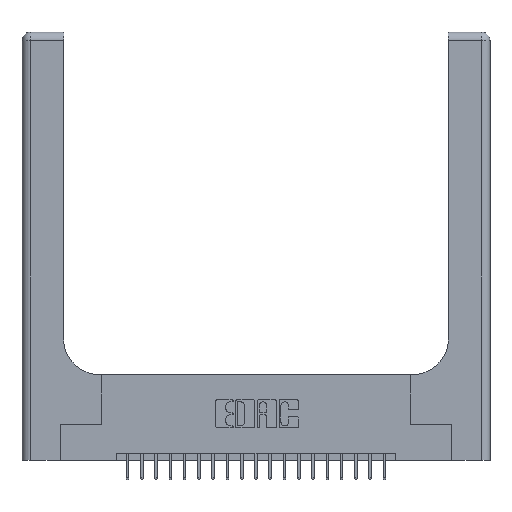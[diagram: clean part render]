
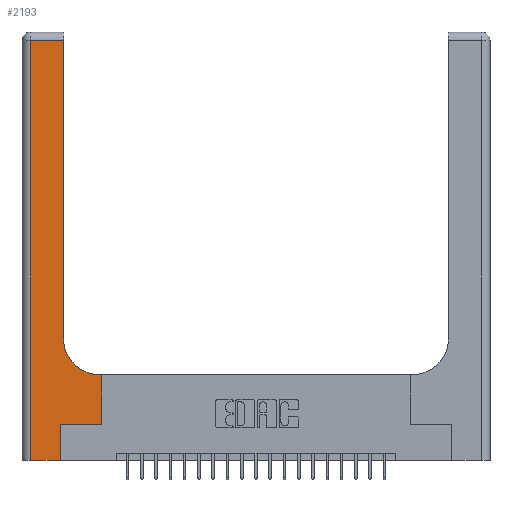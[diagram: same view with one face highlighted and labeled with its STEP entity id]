
A CAD part, top view. The second image highlights one B-rep face of the part: STEP entity #2193.
In plain terms, the highlighted planar face has unit normal (0, 0, 1).
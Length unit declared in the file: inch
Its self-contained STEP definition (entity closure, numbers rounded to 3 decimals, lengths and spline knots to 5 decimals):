
#131 = VECTOR ( 'NONE', #7174, 39.37008 ) ;
#459 = LINE ( 'NONE', #18379, #3451 ) ;
#700 = ORIENTED_EDGE ( 'NONE', *, *, #3910, .T. ) ;
#1152 = CARTESIAN_POINT ( 'NONE',  ( 0.06, 0., 0.37 ) ) ;
#1308 = VECTOR ( 'NONE', #4280, 39.37008 ) ;
#1700 = CARTESIAN_POINT ( 'NONE',  ( 0.2915, 2.94, 0.37 ) ) ;
#2193 = ADVANCED_FACE ( 'NONE', ( #2455 ), #11287, .F. ) ;
#2282 = CARTESIAN_POINT ( 'NONE',  ( 0., 0., 0.37 ) ) ;
#2455 = FACE_OUTER_BOUND ( 'NONE', #15732, .T. ) ;
#2681 = CARTESIAN_POINT ( 'NONE',  ( 0., 3., 0.37 ) ) ;
#2839 = CARTESIAN_POINT ( 'NONE',  ( 0.06, 3., 0.37 ) ) ;
#3423 = VECTOR ( 'NONE', #23259, 39.37008 ) ;
#3451 = VECTOR ( 'NONE', #14610, 39.37008 ) ;
#3501 = LINE ( 'NONE', #17420, #131 ) ;
#3525 = CARTESIAN_POINT ( 'NONE',  ( 0.2915, 0.85, 0.37 ) ) ;
#3741 = VERTEX_POINT ( 'NONE', #12595 ) ;
#3895 = VERTEX_POINT ( 'NONE', #1700 ) ;
#3910 = EDGE_CURVE ( 'NONE', #21596, #21954, #8897, .T. ) ;
#4280 = DIRECTION ( 'NONE',  ( 0., 1., 0. ) ) ;
#5492 = CARTESIAN_POINT ( 'NONE',  ( 0.06, 2.94, 0.37 ) ) ;
#5780 = CARTESIAN_POINT ( 'NONE',  ( 0.269, 0., 0.37 ) ) ;
#7174 = DIRECTION ( 'NONE',  ( 0., 1., 0. ) ) ;
#7654 = DIRECTION ( 'NONE',  ( -1., 0., 0. ) ) ;
#7716 = CARTESIAN_POINT ( 'NONE',  ( 0.2915, 3., 0.37 ) ) ;
#7740 = VECTOR ( 'NONE', #10217, 39.37008 ) ;
#8148 = ORIENTED_EDGE ( 'NONE', *, *, #12432, .T. ) ;
#8198 = VERTEX_POINT ( 'NONE', #3525 ) ;
#8897 = LINE ( 'NONE', #16078, #3423 ) ;
#9439 = DIRECTION ( 'NONE',  ( 0., 0., -1. ) ) ;
#9470 = DIRECTION ( 'NONE',  ( 1., 0., 0. ) ) ;
#9679 = CARTESIAN_POINT ( 'NONE',  ( 0.5415, 0.85, 0.37 ) ) ;
#9809 = ORIENTED_EDGE ( 'NONE', *, *, #11698, .T. ) ;
#10032 = DIRECTION ( 'NONE',  ( 0., -1., 0. ) ) ;
#10217 = DIRECTION ( 'NONE',  ( -1., 0., 0. ) ) ;
#10438 = EDGE_CURVE ( 'NONE', #8198, #3895, #22182, .T. ) ;
#10531 = CARTESIAN_POINT ( 'NONE',  ( 0.5585, 0.6, 0.37 ) ) ;
#10586 = VERTEX_POINT ( 'NONE', #11712 ) ;
#11007 = EDGE_CURVE ( 'NONE', #12067, #10586, #3501, .T. ) ;
#11071 = CIRCLE ( 'NONE', #20100, 0.25 ) ;
#11220 = ORIENTED_EDGE ( 'NONE', *, *, #11007, .T. ) ;
#11287 = PLANE ( 'NONE',  #20291 ) ;
#11392 = CARTESIAN_POINT ( 'NONE',  ( 0.2915, 0.6, 0.37 ) ) ;
#11698 = EDGE_CURVE ( 'NONE', #3741, #8198, #11071, .T. ) ;
#11712 = CARTESIAN_POINT ( 'NONE',  ( 0.269, 0.25, 0.37 ) ) ;
#12067 = VERTEX_POINT ( 'NONE', #5780 ) ;
#12432 = EDGE_CURVE ( 'NONE', #21954, #3741, #20350, .T. ) ;
#12531 = EDGE_CURVE ( 'NONE', #3895, #18633, #22822, .T. ) ;
#12595 = CARTESIAN_POINT ( 'NONE',  ( 0.5415, 0.6, 0.37 ) ) ;
#12934 = ORIENTED_EDGE ( 'NONE', *, *, #18873, .T. ) ;
#14008 = ORIENTED_EDGE ( 'NONE', *, *, #10438, .T. ) ;
#14610 = DIRECTION ( 'NONE',  ( 1., 0., 0. ) ) ;
#14866 = VECTOR ( 'NONE', #16814, 39.37008 ) ;
#15732 = EDGE_LOOP ( 'NONE', ( #14008, #20860, #22919, #12934, #11220, #17727, #700, #8148, #9809 ) ) ;
#16078 = CARTESIAN_POINT ( 'NONE',  ( 0.5585, 0.25, 0.37 ) ) ;
#16448 = EDGE_CURVE ( 'NONE', #18633, #23143, #18991, .T. ) ;
#16635 = DIRECTION ( 'NONE',  ( 1., 0., 0. ) ) ;
#16814 = DIRECTION ( 'NONE',  ( -1., 0., 0. ) ) ;
#16828 = DIRECTION ( 'NONE',  ( 0., 0., -1. ) ) ;
#16939 = VECTOR ( 'NONE', #9470, 39.37008 ) ;
#17420 = CARTESIAN_POINT ( 'NONE',  ( 0.269, 0., 0.37 ) ) ;
#17727 = ORIENTED_EDGE ( 'NONE', *, *, #21395, .T. ) ;
#17976 = VECTOR ( 'NONE', #10032, 39.37008 ) ;
#18379 = CARTESIAN_POINT ( 'NONE',  ( 0.269, 0.25, 0.37 ) ) ;
#18425 = LINE ( 'NONE', #2282, #16939 ) ;
#18633 = VERTEX_POINT ( 'NONE', #5492 ) ;
#18873 = EDGE_CURVE ( 'NONE', #23143, #12067, #18425, .T. ) ;
#18991 = LINE ( 'NONE', #2839, #17976 ) ;
#19164 = CARTESIAN_POINT ( 'NONE',  ( 0., 2.94, 0.37 ) ) ;
#20100 = AXIS2_PLACEMENT_3D ( 'NONE', #9679, #9439, #16635 ) ;
#20291 = AXIS2_PLACEMENT_3D ( 'NONE', #2681, #16828, #7654 ) ;
#20350 = LINE ( 'NONE', #11392, #14866 ) ;
#20860 = ORIENTED_EDGE ( 'NONE', *, *, #12531, .T. ) ;
#21326 = CARTESIAN_POINT ( 'NONE',  ( 0.5585, 0.25, 0.37 ) ) ;
#21395 = EDGE_CURVE ( 'NONE', #10586, #21596, #459, .T. ) ;
#21596 = VERTEX_POINT ( 'NONE', #21326 ) ;
#21954 = VERTEX_POINT ( 'NONE', #10531 ) ;
#22182 = LINE ( 'NONE', #7716, #1308 ) ;
#22822 = LINE ( 'NONE', #19164, #7740 ) ;
#22919 = ORIENTED_EDGE ( 'NONE', *, *, #16448, .T. ) ;
#23143 = VERTEX_POINT ( 'NONE', #1152 ) ;
#23259 = DIRECTION ( 'NONE',  ( 0., 1., 0. ) ) ;
